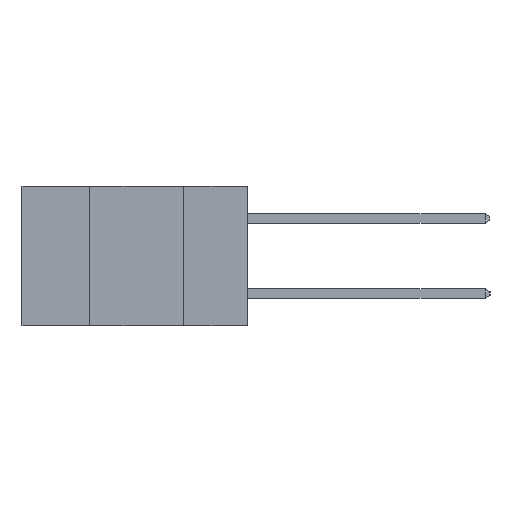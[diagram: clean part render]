
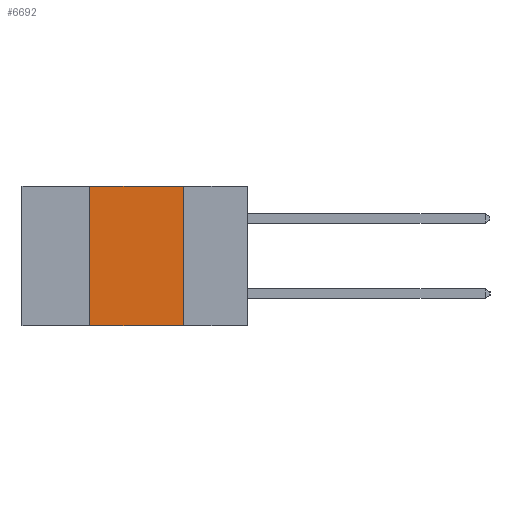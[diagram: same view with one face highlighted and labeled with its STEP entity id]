
A CAD part, left-side view. The second image highlights one B-rep face of the part: STEP entity #6692.
In plain terms, the highlighted planar face has unit normal (-1, 0, 0).
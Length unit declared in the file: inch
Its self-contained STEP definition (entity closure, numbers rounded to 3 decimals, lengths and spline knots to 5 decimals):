
#117 = VERTEX_POINT ( 'NONE', #6757 ) ;
#484 = ORIENTED_EDGE ( 'NONE', *, *, #8593, .F. ) ;
#514 = VERTEX_POINT ( 'NONE', #3373 ) ;
#644 = ORIENTED_EDGE ( 'NONE', *, *, #7020, .F. ) ;
#735 = LINE ( 'NONE', #2275, #6993 ) ;
#1241 = LINE ( 'NONE', #2254, #3217 ) ;
#1532 = CARTESIAN_POINT ( 'NONE',  ( 0., 0.6, -0.37 ) ) ;
#2237 = DIRECTION ( 'NONE',  ( 0., 0., 1. ) ) ;
#2254 = CARTESIAN_POINT ( 'NONE',  ( 0., 0.17, -0.37 ) ) ;
#2275 = CARTESIAN_POINT ( 'NONE',  ( 0., 0.42, -0.37 ) ) ;
#2314 = EDGE_LOOP ( 'NONE', ( #484, #644, #5035, #7653 ) ) ;
#2417 = CARTESIAN_POINT ( 'NONE',  ( 0., 0.42, -0.37 ) ) ;
#2494 = DIRECTION ( 'NONE',  ( 1., 0., 0. ) ) ;
#2921 = CARTESIAN_POINT ( 'NONE',  ( 0., 0.6, 0. ) ) ;
#3217 = VECTOR ( 'NONE', #7057, 39.37008 ) ;
#3301 = CARTESIAN_POINT ( 'NONE',  ( 0., 0.6, 0. ) ) ;
#3373 = CARTESIAN_POINT ( 'NONE',  ( 0., 0.17, -0.37 ) ) ;
#3651 = VECTOR ( 'NONE', #7960, 39.37008 ) ;
#3921 = LINE ( 'NONE', #1532, #3651 ) ;
#5035 = ORIENTED_EDGE ( 'NONE', *, *, #6516, .F. ) ;
#5461 = EDGE_CURVE ( 'NONE', #9894, #514, #3921, .T. ) ;
#5528 = FACE_OUTER_BOUND ( 'NONE', #2314, .T. ) ;
#6158 = DIRECTION ( 'NONE',  ( 0., -1., 0. ) ) ;
#6255 = LINE ( 'NONE', #2921, #8091 ) ;
#6389 = AXIS2_PLACEMENT_3D ( 'NONE', #3301, #2494, #8076 ) ;
#6516 = EDGE_CURVE ( 'NONE', #9894, #9069, #735, .T. ) ;
#6692 = ADVANCED_FACE ( 'NONE', ( #5528 ), #7262, .F. ) ;
#6757 = CARTESIAN_POINT ( 'NONE',  ( 0., 0.17, 0. ) ) ;
#6993 = VECTOR ( 'NONE', #2237, 39.37008 ) ;
#7020 = EDGE_CURVE ( 'NONE', #9069, #117, #6255, .T. ) ;
#7057 = DIRECTION ( 'NONE',  ( 0., 0., -1. ) ) ;
#7262 = PLANE ( 'NONE',  #6389 ) ;
#7584 = CARTESIAN_POINT ( 'NONE',  ( 0., 0.42, 0. ) ) ;
#7653 = ORIENTED_EDGE ( 'NONE', *, *, #5461, .T. ) ;
#7960 = DIRECTION ( 'NONE',  ( 0., -1., 0. ) ) ;
#8076 = DIRECTION ( 'NONE',  ( 0., 0., -1. ) ) ;
#8091 = VECTOR ( 'NONE', #6158, 39.37008 ) ;
#8593 = EDGE_CURVE ( 'NONE', #117, #514, #1241, .T. ) ;
#9069 = VERTEX_POINT ( 'NONE', #7584 ) ;
#9894 = VERTEX_POINT ( 'NONE', #2417 ) ;
